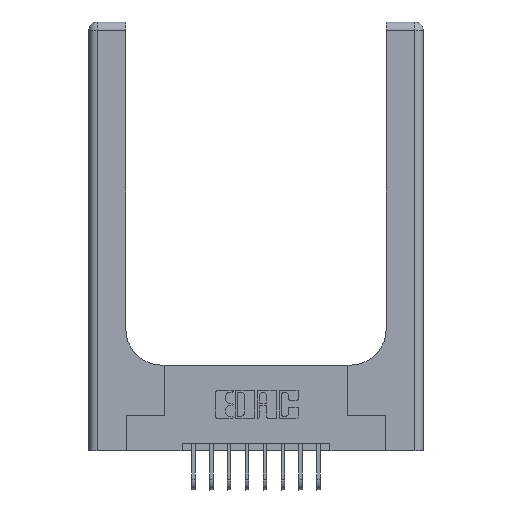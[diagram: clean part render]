
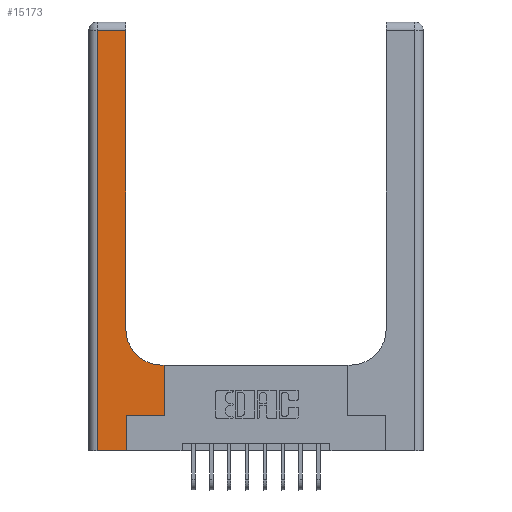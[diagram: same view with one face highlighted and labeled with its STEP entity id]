
A CAD part, top view. The second image highlights one B-rep face of the part: STEP entity #15173.
In plain terms, the highlighted planar face has unit normal (0, 0, 1).
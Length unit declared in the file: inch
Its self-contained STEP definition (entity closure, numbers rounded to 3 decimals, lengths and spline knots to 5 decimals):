
#64 = CARTESIAN_POINT ( 'NONE',  ( 0.265, 0.25, 0.37 ) ) ;
#194 = CARTESIAN_POINT ( 'NONE',  ( 0.06, 3., 0.37 ) ) ;
#428 = CARTESIAN_POINT ( 'NONE',  ( 0.51, 0.85, 0.37 ) ) ;
#690 = VECTOR ( 'NONE', #1833, 39.37008 ) ;
#1000 = EDGE_CURVE ( 'NONE', #14150, #14142, #11663, .T. ) ;
#1318 = VERTEX_POINT ( 'NONE', #16190 ) ;
#1319 = VECTOR ( 'NONE', #11609, 39.37008 ) ;
#1534 = LINE ( 'NONE', #5361, #2047 ) ;
#1657 = CARTESIAN_POINT ( 'NONE',  ( 0.26, 2.94, 0.37 ) ) ;
#1833 = DIRECTION ( 'NONE',  ( 0., 1., 0. ) ) ;
#2047 = VECTOR ( 'NONE', #15907, 39.37008 ) ;
#2268 = ORIENTED_EDGE ( 'NONE', *, *, #1000, .T. ) ;
#2270 = ORIENTED_EDGE ( 'NONE', *, *, #12224, .T. ) ;
#2551 = LINE ( 'NONE', #11827, #3859 ) ;
#2737 = LINE ( 'NONE', #194, #12872 ) ;
#2832 = VERTEX_POINT ( 'NONE', #14606 ) ;
#2933 = AXIS2_PLACEMENT_3D ( 'NONE', #428, #4514, #9822 ) ;
#2993 = DIRECTION ( 'NONE',  ( 0., -1., 0. ) ) ;
#3164 = ORIENTED_EDGE ( 'NONE', *, *, #10947, .T. ) ;
#3598 = DIRECTION ( 'NONE',  ( -1., 0., 0. ) ) ;
#3859 = VECTOR ( 'NONE', #6799, 39.37008 ) ;
#4226 = LINE ( 'NONE', #9527, #12141 ) ;
#4291 = LINE ( 'NONE', #9773, #13516 ) ;
#4514 = DIRECTION ( 'NONE',  ( 0., 0., -1. ) ) ;
#4535 = EDGE_CURVE ( 'NONE', #2832, #10118, #1534, .T. ) ;
#4882 = DIRECTION ( 'NONE',  ( 0., 0., -1. ) ) ;
#5078 = EDGE_CURVE ( 'NONE', #6535, #14150, #4226, .T. ) ;
#5361 = CARTESIAN_POINT ( 'NONE',  ( 0.26, 3., 0.37 ) ) ;
#5690 = CIRCLE ( 'NONE', #2933, 0.25 ) ;
#5853 = ORIENTED_EDGE ( 'NONE', *, *, #5078, .T. ) ;
#5868 = VECTOR ( 'NONE', #15349, 39.37008 ) ;
#6189 = FACE_OUTER_BOUND ( 'NONE', #9841, .T. ) ;
#6227 = AXIS2_PLACEMENT_3D ( 'NONE', #16812, #4882, #3598 ) ;
#6535 = VERTEX_POINT ( 'NONE', #13152 ) ;
#6799 = DIRECTION ( 'NONE',  ( 1., 0., 0. ) ) ;
#7069 = DIRECTION ( 'NONE',  ( -1., 0., 0. ) ) ;
#8772 = VERTEX_POINT ( 'NONE', #64 ) ;
#8784 = ORIENTED_EDGE ( 'NONE', *, *, #9765, .T. ) ;
#9527 = CARTESIAN_POINT ( 'NONE',  ( 0.528, 0.25, 0.37 ) ) ;
#9637 = CARTESIAN_POINT ( 'NONE',  ( 0.528, 0.6, 0.37 ) ) ;
#9765 = EDGE_CURVE ( 'NONE', #10118, #1318, #4291, .T. ) ;
#9773 = CARTESIAN_POINT ( 'NONE',  ( 0., 2.94, 0.37 ) ) ;
#9822 = DIRECTION ( 'NONE',  ( 1., 0., 0. ) ) ;
#9841 = EDGE_LOOP ( 'NONE', ( #11161, #8784, #14200, #2270, #10425, #3164, #5853, #2268, #10286 ) ) ;
#10118 = VERTEX_POINT ( 'NONE', #1657 ) ;
#10286 = ORIENTED_EDGE ( 'NONE', *, *, #16645, .T. ) ;
#10322 = LINE ( 'NONE', #15716, #1319 ) ;
#10425 = ORIENTED_EDGE ( 'NONE', *, *, #13665, .T. ) ;
#10776 = CARTESIAN_POINT ( 'NONE',  ( 0.265, 0., 0.37 ) ) ;
#10947 = EDGE_CURVE ( 'NONE', #8772, #6535, #2551, .T. ) ;
#11034 = VERTEX_POINT ( 'NONE', #13165 ) ;
#11161 = ORIENTED_EDGE ( 'NONE', *, *, #4535, .T. ) ;
#11478 = PLANE ( 'NONE',  #6227 ) ;
#11485 = CARTESIAN_POINT ( 'NONE',  ( 0.26, 0.6, 0.37 ) ) ;
#11609 = DIRECTION ( 'NONE',  ( 1., 0., 0. ) ) ;
#11663 = LINE ( 'NONE', #11485, #5868 ) ;
#11729 = VERTEX_POINT ( 'NONE', #10776 ) ;
#11827 = CARTESIAN_POINT ( 'NONE',  ( 0.265, 0.25, 0.37 ) ) ;
#12141 = VECTOR ( 'NONE', #13772, 39.37008 ) ;
#12224 = EDGE_CURVE ( 'NONE', #11034, #11729, #10322, .T. ) ;
#12872 = VECTOR ( 'NONE', #2993, 39.37008 ) ;
#13152 = CARTESIAN_POINT ( 'NONE',  ( 0.528, 0.25, 0.37 ) ) ;
#13165 = CARTESIAN_POINT ( 'NONE',  ( 0.06, 0., 0.37 ) ) ;
#13516 = VECTOR ( 'NONE', #7069, 39.37008 ) ;
#13665 = EDGE_CURVE ( 'NONE', #11729, #8772, #13819, .T. ) ;
#13772 = DIRECTION ( 'NONE',  ( 0., 1., 0. ) ) ;
#13819 = LINE ( 'NONE', #16178, #690 ) ;
#14142 = VERTEX_POINT ( 'NONE', #15112 ) ;
#14150 = VERTEX_POINT ( 'NONE', #9637 ) ;
#14200 = ORIENTED_EDGE ( 'NONE', *, *, #14796, .T. ) ;
#14606 = CARTESIAN_POINT ( 'NONE',  ( 0.26, 0.85, 0.37 ) ) ;
#14796 = EDGE_CURVE ( 'NONE', #1318, #11034, #2737, .T. ) ;
#15112 = CARTESIAN_POINT ( 'NONE',  ( 0.51, 0.6, 0.37 ) ) ;
#15173 = ADVANCED_FACE ( 'NONE', ( #6189 ), #11478, .F. ) ;
#15349 = DIRECTION ( 'NONE',  ( -1., 0., 0. ) ) ;
#15716 = CARTESIAN_POINT ( 'NONE',  ( 0., 0., 0.37 ) ) ;
#15907 = DIRECTION ( 'NONE',  ( 0., 1., 0. ) ) ;
#16178 = CARTESIAN_POINT ( 'NONE',  ( 0.265, 0., 0.37 ) ) ;
#16190 = CARTESIAN_POINT ( 'NONE',  ( 0.06, 2.94, 0.37 ) ) ;
#16645 = EDGE_CURVE ( 'NONE', #14142, #2832, #5690, .T. ) ;
#16812 = CARTESIAN_POINT ( 'NONE',  ( 0., 3., 0.37 ) ) ;
